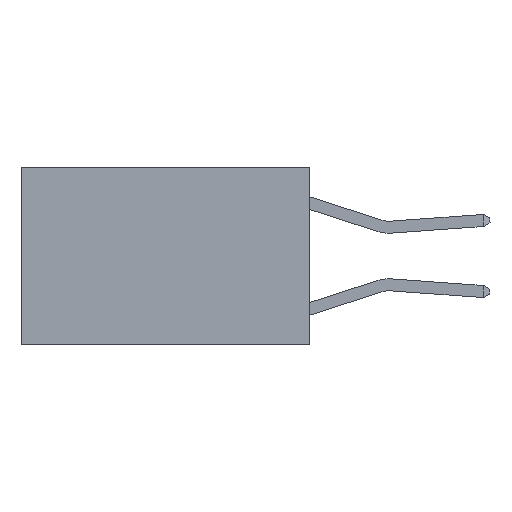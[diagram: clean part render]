
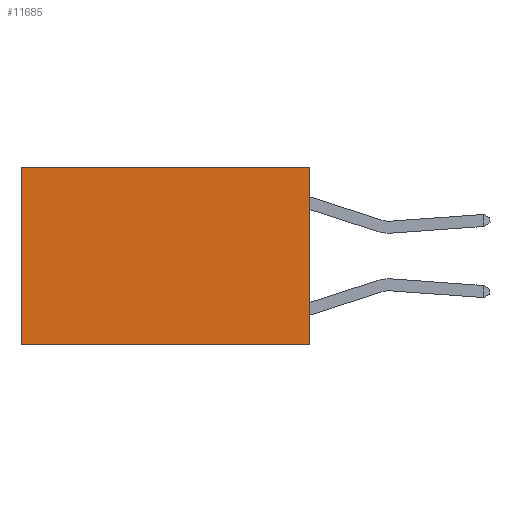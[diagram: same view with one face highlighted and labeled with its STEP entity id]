
A CAD part, left-side view. The second image highlights one B-rep face of the part: STEP entity #11685.
In plain terms, the highlighted planar face has unit normal (-1, 0, 0).
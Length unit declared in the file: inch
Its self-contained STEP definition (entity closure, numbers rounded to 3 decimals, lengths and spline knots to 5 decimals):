
#1165 = CARTESIAN_POINT ( 'NONE',  ( 0.2625, 0., -0.37 ) ) ;
#1350 = VERTEX_POINT ( 'NONE', #5612 ) ;
#2045 = DIRECTION ( 'NONE',  ( 0., 1., 0. ) ) ;
#2087 = VECTOR ( 'NONE', #10239, 39.37008 ) ;
#2533 = CARTESIAN_POINT ( 'NONE',  ( 0.2625, 0., 0. ) ) ;
#3123 = FACE_OUTER_BOUND ( 'NONE', #3439, .T. ) ;
#3439 = EDGE_LOOP ( 'NONE', ( #3803, #8125, #9505, #4102 ) ) ;
#3509 = AXIS2_PLACEMENT_3D ( 'NONE', #2533, #12742, #6566 ) ;
#3803 = ORIENTED_EDGE ( 'NONE', *, *, #4858, .T. ) ;
#4102 = ORIENTED_EDGE ( 'NONE', *, *, #5873, .T. ) ;
#4472 = VECTOR ( 'NONE', #4833, 39.37008 ) ;
#4833 = DIRECTION ( 'NONE',  ( 0., 0., -1. ) ) ;
#4858 = EDGE_CURVE ( 'NONE', #6912, #5684, #9471, .T. ) ;
#4889 = CARTESIAN_POINT ( 'NONE',  ( 0.2625, 0., 0. ) ) ;
#5612 = CARTESIAN_POINT ( 'NONE',  ( 0.2625, 0., 0. ) ) ;
#5684 = VERTEX_POINT ( 'NONE', #8383 ) ;
#5711 = CARTESIAN_POINT ( 'NONE',  ( 0.2625, 0.6, 0. ) ) ;
#5873 = EDGE_CURVE ( 'NONE', #1350, #6912, #12809, .T. ) ;
#6566 = DIRECTION ( 'NONE',  ( 0., 0., -1. ) ) ;
#6906 = DIRECTION ( 'NONE',  ( 0., 1., 0. ) ) ;
#6912 = VERTEX_POINT ( 'NONE', #5711 ) ;
#8125 = ORIENTED_EDGE ( 'NONE', *, *, #10650, .F. ) ;
#8295 = CARTESIAN_POINT ( 'NONE',  ( 0.2625, 0., -0.37 ) ) ;
#8383 = CARTESIAN_POINT ( 'NONE',  ( 0.2625, 0.6, -0.37 ) ) ;
#8448 = EDGE_CURVE ( 'NONE', #1350, #10603, #10592, .T. ) ;
#9471 = LINE ( 'NONE', #12953, #4472 ) ;
#9505 = ORIENTED_EDGE ( 'NONE', *, *, #8448, .F. ) ;
#9594 = VECTOR ( 'NONE', #6906, 39.37008 ) ;
#10239 = DIRECTION ( 'NONE',  ( 0., 0., -1. ) ) ;
#10592 = LINE ( 'NONE', #12264, #2087 ) ;
#10603 = VERTEX_POINT ( 'NONE', #8295 ) ;
#10650 = EDGE_CURVE ( 'NONE', #10603, #5684, #11518, .T. ) ;
#11518 = LINE ( 'NONE', #1165, #12641 ) ;
#11685 = ADVANCED_FACE ( 'NONE', ( #3123 ), #11790, .F. ) ;
#11790 = PLANE ( 'NONE',  #3509 ) ;
#12264 = CARTESIAN_POINT ( 'NONE',  ( 0.2625, 0., 0. ) ) ;
#12641 = VECTOR ( 'NONE', #2045, 39.37008 ) ;
#12742 = DIRECTION ( 'NONE',  ( 1., 0., 0. ) ) ;
#12809 = LINE ( 'NONE', #4889, #9594 ) ;
#12953 = CARTESIAN_POINT ( 'NONE',  ( 0.2625, 0.6, 0. ) ) ;
